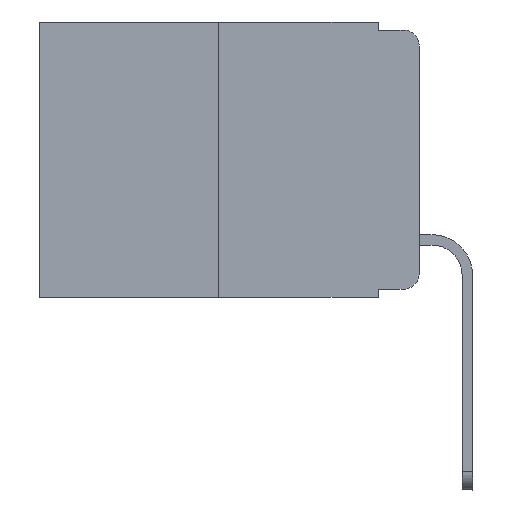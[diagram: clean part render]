
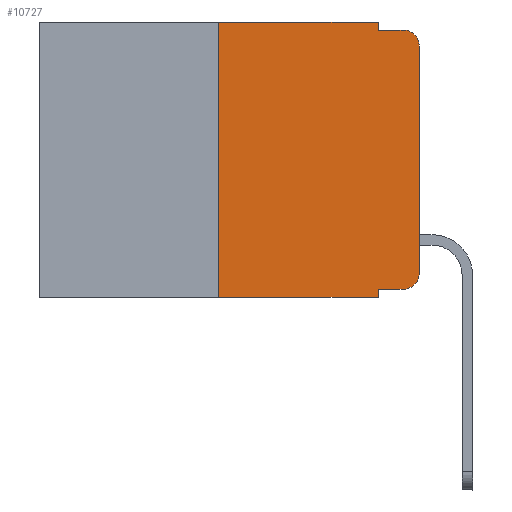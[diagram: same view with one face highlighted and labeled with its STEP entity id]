
A CAD part, left-side view. The second image highlights one B-rep face of the part: STEP entity #10727.
In plain terms, the highlighted planar face has unit normal (-1, 0, 0).
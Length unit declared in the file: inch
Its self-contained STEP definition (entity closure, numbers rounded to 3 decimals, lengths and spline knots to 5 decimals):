
#231 = EDGE_CURVE ( 'NONE', #7915, #2458, #8479, .T. ) ;
#428 = CARTESIAN_POINT ( 'NONE',  ( 0., 0.02, -0.333 ) ) ;
#597 = VERTEX_POINT ( 'NONE', #12694 ) ;
#788 = CARTESIAN_POINT ( 'NONE',  ( 0., 0.051, 0. ) ) ;
#807 = EDGE_CURVE ( 'NONE', #7915, #7414, #9386, .T. ) ;
#1139 = LINE ( 'NONE', #6334, #2030 ) ;
#1146 = LINE ( 'NONE', #7225, #7626 ) ;
#1215 = FACE_OUTER_BOUND ( 'NONE', #5612, .T. ) ;
#1391 = DIRECTION ( 'NONE',  ( -1., 0., 0. ) ) ;
#1472 = CARTESIAN_POINT ( 'NONE',  ( 0., 0.473, 0. ) ) ;
#1736 = LINE ( 'NONE', #12948, #5884 ) ;
#1751 = VECTOR ( 'NONE', #12827, 39.37008 ) ;
#1791 = CARTESIAN_POINT ( 'NONE',  ( 0., 0.25, 0. ) ) ;
#2030 = VECTOR ( 'NONE', #5248, 39.37008 ) ;
#2239 = CIRCLE ( 'NONE', #5905, 0.02 ) ;
#2307 = CARTESIAN_POINT ( 'NONE',  ( 0., 0.051, -0.01 ) ) ;
#2406 = CIRCLE ( 'NONE', #9763, 0.02 ) ;
#2458 = VERTEX_POINT ( 'NONE', #6004 ) ;
#2538 = CARTESIAN_POINT ( 'NONE',  ( 0., 0.25, -0.343 ) ) ;
#2598 = DIRECTION ( 'NONE',  ( 0., 0., -1. ) ) ;
#2670 = DIRECTION ( 'NONE',  ( 0., -1., 0. ) ) ;
#2709 = EDGE_CURVE ( 'NONE', #11554, #5861, #1146, .T. ) ;
#3316 = VERTEX_POINT ( 'NONE', #10915 ) ;
#3327 = DIRECTION ( 'NONE',  ( 0., -1., 0. ) ) ;
#3457 = VECTOR ( 'NONE', #8501, 39.37008 ) ;
#3565 = DIRECTION ( 'NONE',  ( 0., 0., -1. ) ) ;
#3604 = DIRECTION ( 'NONE',  ( -1., 0., 0. ) ) ;
#4369 = CARTESIAN_POINT ( 'NONE',  ( 0., 0.25, 0. ) ) ;
#4417 = LINE ( 'NONE', #8546, #6086 ) ;
#5248 = DIRECTION ( 'NONE',  ( 0., 0., -1. ) ) ;
#5257 = DIRECTION ( 'NONE',  ( 0., -1., 0. ) ) ;
#5612 = EDGE_LOOP ( 'NONE', ( #11105, #11176, #10100, #12426, #6355, #10925, #6595, #10662, #7778, #10273 ) ) ;
#5861 = VERTEX_POINT ( 'NONE', #6388 ) ;
#5884 = VECTOR ( 'NONE', #2670, 39.37008 ) ;
#5905 = AXIS2_PLACEMENT_3D ( 'NONE', #9582, #1391, #11663 ) ;
#6004 = CARTESIAN_POINT ( 'NONE',  ( 0., 0.051, -0.343 ) ) ;
#6086 = VECTOR ( 'NONE', #6377, 39.37008 ) ;
#6096 = CARTESIAN_POINT ( 'NONE',  ( 0., 0.051, 0. ) ) ;
#6334 = CARTESIAN_POINT ( 'NONE',  ( 0., 0.051, 0. ) ) ;
#6355 = ORIENTED_EDGE ( 'NONE', *, *, #8701, .F. ) ;
#6377 = DIRECTION ( 'NONE',  ( 0., -1., 0. ) ) ;
#6388 = CARTESIAN_POINT ( 'NONE',  ( 0., 0.02, -0.01 ) ) ;
#6539 = LINE ( 'NONE', #8335, #1751 ) ;
#6595 = ORIENTED_EDGE ( 'NONE', *, *, #231, .T. ) ;
#7225 = CARTESIAN_POINT ( 'NONE',  ( 0., 0.051, -0.01 ) ) ;
#7414 = VERTEX_POINT ( 'NONE', #1791 ) ;
#7626 = VECTOR ( 'NONE', #5257, 39.37008 ) ;
#7778 = ORIENTED_EDGE ( 'NONE', *, *, #9457, .T. ) ;
#7906 = EDGE_CURVE ( 'NONE', #7993, #3316, #6539, .T. ) ;
#7915 = VERTEX_POINT ( 'NONE', #2538 ) ;
#7993 = VERTEX_POINT ( 'NONE', #11073 ) ;
#8335 = CARTESIAN_POINT ( 'NONE',  ( 0., 0., 0. ) ) ;
#8479 = LINE ( 'NONE', #12593, #12265 ) ;
#8501 = DIRECTION ( 'NONE',  ( 0., 0., 1. ) ) ;
#8519 = VECTOR ( 'NONE', #2598, 39.37008 ) ;
#8546 = CARTESIAN_POINT ( 'NONE',  ( 0., 0.473, 0. ) ) ;
#8701 = EDGE_CURVE ( 'NONE', #7414, #8963, #4417, .T. ) ;
#8717 = DIRECTION ( 'NONE',  ( 1., 0., 0. ) ) ;
#8764 = CARTESIAN_POINT ( 'NONE',  ( 0., 0.02, -0.03 ) ) ;
#8822 = VERTEX_POINT ( 'NONE', #428 ) ;
#8963 = VERTEX_POINT ( 'NONE', #6096 ) ;
#9386 = LINE ( 'NONE', #4369, #3457 ) ;
#9457 = EDGE_CURVE ( 'NONE', #597, #8822, #1736, .T. ) ;
#9582 = CARTESIAN_POINT ( 'NONE',  ( 0., 0.02, -0.313 ) ) ;
#9763 = AXIS2_PLACEMENT_3D ( 'NONE', #8764, #3604, #9832 ) ;
#9832 = DIRECTION ( 'NONE',  ( 0., 0., -1. ) ) ;
#10043 = LINE ( 'NONE', #788, #8519 ) ;
#10100 = ORIENTED_EDGE ( 'NONE', *, *, #2709, .F. ) ;
#10142 = EDGE_CURVE ( 'NONE', #3316, #5861, #2406, .T. ) ;
#10273 = ORIENTED_EDGE ( 'NONE', *, *, #12405, .T. ) ;
#10662 = ORIENTED_EDGE ( 'NONE', *, *, #12277, .F. ) ;
#10727 = ADVANCED_FACE ( 'NONE', ( #1215 ), #10740, .F. ) ;
#10740 = PLANE ( 'NONE',  #11915 ) ;
#10915 = CARTESIAN_POINT ( 'NONE',  ( 0., 0., -0.03 ) ) ;
#10925 = ORIENTED_EDGE ( 'NONE', *, *, #807, .F. ) ;
#11073 = CARTESIAN_POINT ( 'NONE',  ( 0., 0., -0.313 ) ) ;
#11105 = ORIENTED_EDGE ( 'NONE', *, *, #7906, .T. ) ;
#11176 = ORIENTED_EDGE ( 'NONE', *, *, #10142, .T. ) ;
#11554 = VERTEX_POINT ( 'NONE', #2307 ) ;
#11663 = DIRECTION ( 'NONE',  ( 0., 0., -1. ) ) ;
#11915 = AXIS2_PLACEMENT_3D ( 'NONE', #1472, #8717, #3565 ) ;
#12265 = VECTOR ( 'NONE', #3327, 39.37008 ) ;
#12277 = EDGE_CURVE ( 'NONE', #597, #2458, #1139, .T. ) ;
#12405 = EDGE_CURVE ( 'NONE', #8822, #7993, #2239, .T. ) ;
#12426 = ORIENTED_EDGE ( 'NONE', *, *, #12647, .F. ) ;
#12593 = CARTESIAN_POINT ( 'NONE',  ( 0., 0.473, -0.343 ) ) ;
#12647 = EDGE_CURVE ( 'NONE', #8963, #11554, #10043, .T. ) ;
#12694 = CARTESIAN_POINT ( 'NONE',  ( 0., 0.051, -0.333 ) ) ;
#12827 = DIRECTION ( 'NONE',  ( 0., 0., 1. ) ) ;
#12948 = CARTESIAN_POINT ( 'NONE',  ( 0., 0.051, -0.333 ) ) ;
